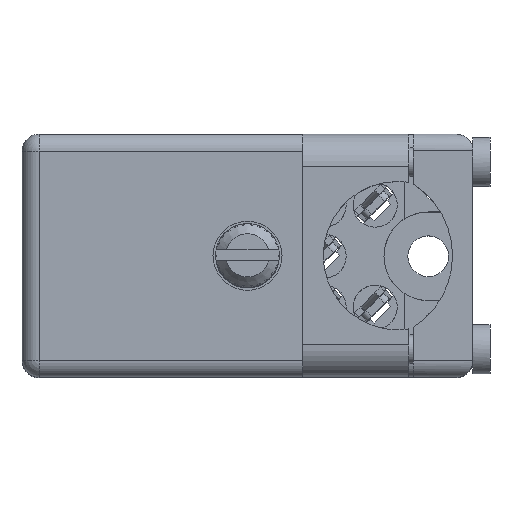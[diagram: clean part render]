
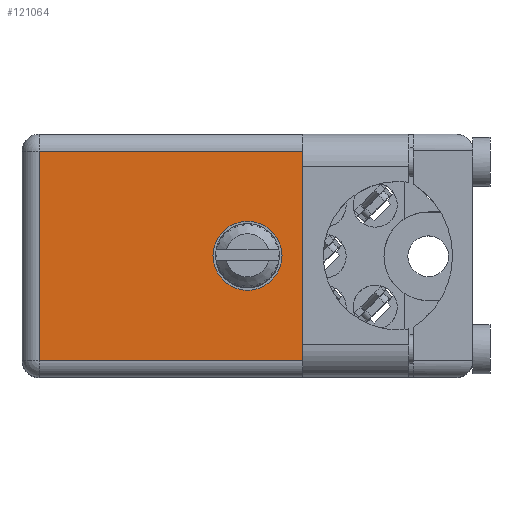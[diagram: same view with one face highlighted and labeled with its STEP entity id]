
A CAD part, top view. The second image highlights one B-rep face of the part: STEP entity #121064.
In plain terms, the highlighted face is planar.
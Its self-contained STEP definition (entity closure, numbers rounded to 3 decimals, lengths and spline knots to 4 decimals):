
#1166 = DIRECTION ( 'NONE',  ( 0., 0., 1. ) ) ;
#1904 = EDGE_CURVE ( 'NONE', #68956, #116942, #73683, .T. ) ;
#3461 = LINE ( 'NONE', #134582, #18458 ) ;
#4244 = CARTESIAN_POINT ( 'NONE',  ( 1.15, 0.906, -0.715 ) ) ;
#7748 = EDGE_CURVE ( 'NONE', #52993, #171332, #103295, .T. ) ;
#10765 = VECTOR ( 'NONE', #42094, 39.3701 ) ;
#14081 = CARTESIAN_POINT ( 'NONE',  ( 0.6625, 0.906, -0.459 ) ) ;
#17227 = DIRECTION ( 'NONE',  ( -1., 0., 0. ) ) ;
#18458 = VECTOR ( 'NONE', #104664, 39.3701 ) ;
#18608 = VERTEX_POINT ( 'NONE', #111310 ) ;
#20454 = CARTESIAN_POINT ( 'NONE',  ( 1.15, 0.906, -0.05 ) ) ;
#21378 = LINE ( 'NONE', #51293, #127252 ) ;
#22553 = AXIS2_PLACEMENT_3D ( 'NONE', #31868, #89887, #32775 ) ;
#24125 = ORIENTED_EDGE ( 'NONE', *, *, #133499, .T. ) ;
#28274 = AXIS2_PLACEMENT_3D ( 'NONE', #77605, #161008, #161937 ) ;
#28491 = EDGE_CURVE ( 'NONE', #181556, #157033, #43022, .T. ) ;
#28630 = CIRCLE ( 'NONE', #181209, 0.1015 ) ;
#30280 = DIRECTION ( 'NONE',  ( 0., 1., 0. ) ) ;
#31510 = DIRECTION ( 'NONE',  ( 0., 0., 1. ) ) ;
#31868 = CARTESIAN_POINT ( 'NONE',  ( 0.6625, 0.906, -0.3575 ) ) ;
#32775 = DIRECTION ( 'NONE',  ( 0., 0., 1. ) ) ;
#36165 = ORIENTED_EDGE ( 'NONE', *, *, #91959, .T. ) ;
#38269 = CARTESIAN_POINT ( 'NONE',  ( 0.05, 0.906, -0.05 ) ) ;
#41149 = CARTESIAN_POINT ( 'NONE',  ( 0.05, 0.906, -0.715 ) ) ;
#42094 = DIRECTION ( 'NONE',  ( 0., 0., 1. ) ) ;
#42467 = VERTEX_POINT ( 'NONE', #124463 ) ;
#43022 = LINE ( 'NONE', #41149, #10765 ) ;
#46155 = DIRECTION ( 'NONE',  ( 0., 0., -1. ) ) ;
#48135 = EDGE_CURVE ( 'NONE', #50163, #18608, #3461, .T. ) ;
#50163 = VERTEX_POINT ( 'NONE', #181284 ) ;
#51293 = CARTESIAN_POINT ( 'NONE',  ( 0.865, 0.906, -0.6025 ) ) ;
#52993 = VERTEX_POINT ( 'NONE', #14081 ) ;
#60290 = CARTESIAN_POINT ( 'NONE',  ( 0.865, 0.906, -0.1125 ) ) ;
#68956 = VERTEX_POINT ( 'NONE', #140411 ) ;
#69279 = ORIENTED_EDGE ( 'NONE', *, *, #48135, .F. ) ;
#73683 = LINE ( 'NONE', #4244, #85135 ) ;
#74840 = FACE_OUTER_BOUND ( 'NONE', #133436, .T. ) ;
#77605 = CARTESIAN_POINT ( 'NONE',  ( 0., 0.906, -0.715 ) ) ;
#78484 = DIRECTION ( 'NONE',  ( 1., 0., 0. ) ) ;
#78769 = VECTOR ( 'NONE', #46155, 39.3701 ) ;
#83078 = ORIENTED_EDGE ( 'NONE', *, *, #7748, .F. ) ;
#85135 = VECTOR ( 'NONE', #31510, 39.3701 ) ;
#89887 = DIRECTION ( 'NONE',  ( 0., 1., 0. ) ) ;
#91439 = EDGE_LOOP ( 'NONE', ( #135042, #83078 ) ) ;
#91664 = PLANE ( 'NONE',  #28274 ) ;
#91959 = EDGE_CURVE ( 'NONE', #50163, #116775, #116499, .T. ) ;
#102974 = VECTOR ( 'NONE', #163748, 39.3701 ) ;
#103295 = CIRCLE ( 'NONE', #22553, 0.1015 ) ;
#103997 = EDGE_CURVE ( 'NONE', #116775, #42467, #185141, .T. ) ;
#104664 = DIRECTION ( 'NONE',  ( 0., 0., 1. ) ) ;
#109275 = EDGE_CURVE ( 'NONE', #157033, #18608, #120611, .T. ) ;
#111310 = CARTESIAN_POINT ( 'NONE',  ( 1.15, 0.906, -0.05 ) ) ;
#116499 = LINE ( 'NONE', #60290, #157371 ) ;
#116775 = VERTEX_POINT ( 'NONE', #129379 ) ;
#116942 = VERTEX_POINT ( 'NONE', #145329 ) ;
#117330 = CARTESIAN_POINT ( 'NONE',  ( 0.865, 0.906, -0.1125 ) ) ;
#120611 = LINE ( 'NONE', #20454, #102974 ) ;
#121064 = ADVANCED_FACE ( 'NONE', ( #74840, #131929 ), #91664, .T. ) ;
#121435 = LINE ( 'NONE', #177689, #156504 ) ;
#124463 = CARTESIAN_POINT ( 'NONE',  ( 0.865, 0.906, -0.6025 ) ) ;
#127252 = VECTOR ( 'NONE', #78484, 39.3701 ) ;
#128497 = CARTESIAN_POINT ( 'NONE',  ( 0.05, 0.906, -0.665 ) ) ;
#129379 = CARTESIAN_POINT ( 'NONE',  ( 0.865, 0.906, -0.1125 ) ) ;
#131929 = FACE_BOUND ( 'NONE', #91439, .T. ) ;
#133436 = EDGE_LOOP ( 'NONE', ( #133662, #134884, #69279, #36165, #169392, #155613, #134677, #24125 ) ) ;
#133499 = EDGE_CURVE ( 'NONE', #68956, #181556, #121435, .T. ) ;
#133662 = ORIENTED_EDGE ( 'NONE', *, *, #28491, .T. ) ;
#134582 = CARTESIAN_POINT ( 'NONE',  ( 1.15, 0.906, -0.715 ) ) ;
#134677 = ORIENTED_EDGE ( 'NONE', *, *, #1904, .F. ) ;
#134884 = ORIENTED_EDGE ( 'NONE', *, *, #109275, .T. ) ;
#135042 = ORIENTED_EDGE ( 'NONE', *, *, #172042, .F. ) ;
#140411 = CARTESIAN_POINT ( 'NONE',  ( 1.15, 0.906, -0.665 ) ) ;
#145329 = CARTESIAN_POINT ( 'NONE',  ( 1.15, 0.906, -0.6025 ) ) ;
#155613 = ORIENTED_EDGE ( 'NONE', *, *, #180549, .T. ) ;
#156504 = VECTOR ( 'NONE', #178627, 39.3701 ) ;
#156731 = CARTESIAN_POINT ( 'NONE',  ( 0.6625, 0.906, -0.3575 ) ) ;
#157033 = VERTEX_POINT ( 'NONE', #38269 ) ;
#157371 = VECTOR ( 'NONE', #17227, 39.3701 ) ;
#161008 = DIRECTION ( 'NONE',  ( 0., 1., 0. ) ) ;
#161937 = DIRECTION ( 'NONE',  ( 0., 0., 1. ) ) ;
#162465 = CARTESIAN_POINT ( 'NONE',  ( 0.6625, 0.906, -0.256 ) ) ;
#163748 = DIRECTION ( 'NONE',  ( 1., 0., 0. ) ) ;
#169392 = ORIENTED_EDGE ( 'NONE', *, *, #103997, .T. ) ;
#171332 = VERTEX_POINT ( 'NONE', #162465 ) ;
#172042 = EDGE_CURVE ( 'NONE', #171332, #52993, #28630, .T. ) ;
#177689 = CARTESIAN_POINT ( 'NONE',  ( 0., 0.906, -0.665 ) ) ;
#178627 = DIRECTION ( 'NONE',  ( -1., 0., 0. ) ) ;
#180549 = EDGE_CURVE ( 'NONE', #42467, #116942, #21378, .T. ) ;
#181209 = AXIS2_PLACEMENT_3D ( 'NONE', #156731, #30280, #1166 ) ;
#181284 = CARTESIAN_POINT ( 'NONE',  ( 1.15, 0.906, -0.1125 ) ) ;
#181556 = VERTEX_POINT ( 'NONE', #128497 ) ;
#185141 = LINE ( 'NONE', #117330, #78769 ) ;
